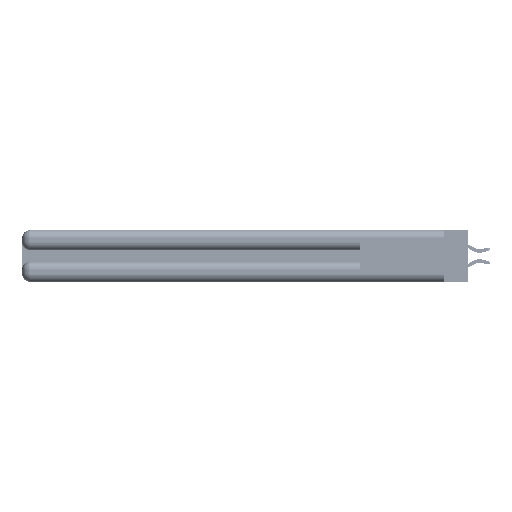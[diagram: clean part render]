
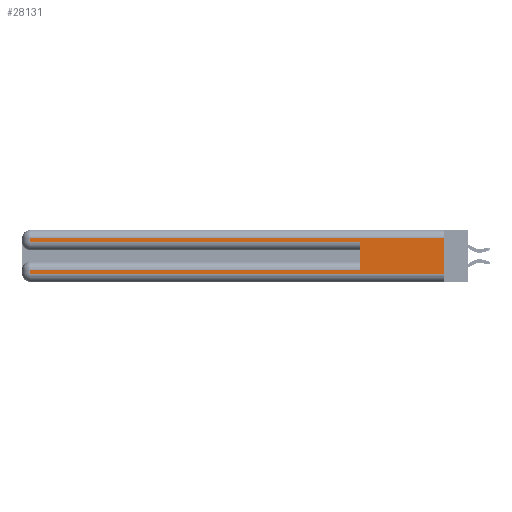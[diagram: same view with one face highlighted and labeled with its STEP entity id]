
A CAD part, left-side view. The second image highlights one B-rep face of the part: STEP entity #28131.
In plain terms, the highlighted planar face has unit normal (-1, 0, 0).
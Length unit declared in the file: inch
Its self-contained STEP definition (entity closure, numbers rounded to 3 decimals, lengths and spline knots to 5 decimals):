
#3 = EDGE_LOOP ( 'NONE', ( #18414, #37219, #32629, #33383, #12969, #47455, #42234, #39631 ) ) ;
#504 = EDGE_CURVE ( 'NONE', #51900, #22637, #47891, .T. ) ;
#625 = VECTOR ( 'NONE', #6461, 39.37008 ) ;
#2067 = LINE ( 'NONE', #34609, #21926 ) ;
#4163 = EDGE_CURVE ( 'NONE', #12128, #20755, #49559, .T. ) ;
#4641 = VECTOR ( 'NONE', #5702, 39.37008 ) ;
#5702 = DIRECTION ( 'NONE',  ( 0., 1., 0. ) ) ;
#6461 = DIRECTION ( 'NONE',  ( 0., 0., -1. ) ) ;
#8053 = EDGE_CURVE ( 'NONE', #45056, #49565, #25386, .T. ) ;
#8858 = CARTESIAN_POINT ( 'NONE',  ( 0., 0.6, 0.285 ) ) ;
#8896 = LINE ( 'NONE', #9161, #18818 ) ;
#9161 = CARTESIAN_POINT ( 'NONE',  ( 0., 2.94, 0.37 ) ) ;
#10229 = CARTESIAN_POINT ( 'NONE',  ( 0., 0., 0.085 ) ) ;
#11843 = CARTESIAN_POINT ( 'NONE',  ( 0., 0., 0.37 ) ) ;
#11967 = LINE ( 'NONE', #36004, #625 ) ;
#12128 = VERTEX_POINT ( 'NONE', #51677 ) ;
#12969 = ORIENTED_EDGE ( 'NONE', *, *, #20425, .F. ) ;
#14030 = EDGE_CURVE ( 'NONE', #29570, #34548, #2067, .T. ) ;
#14033 = CARTESIAN_POINT ( 'NONE',  ( 0., 0., 0.31 ) ) ;
#14409 = CARTESIAN_POINT ( 'NONE',  ( 0., 0.6, 0.145 ) ) ;
#16078 = DIRECTION ( 'NONE',  ( 0., 0., -1. ) ) ;
#16419 = CARTESIAN_POINT ( 'NONE',  ( 0., 2.94, 0.31 ) ) ;
#16891 = FACE_OUTER_BOUND ( 'NONE', #3, .T. ) ;
#17094 = CARTESIAN_POINT ( 'NONE',  ( 0., 0., 0.37 ) ) ;
#18414 = ORIENTED_EDGE ( 'NONE', *, *, #40958, .F. ) ;
#18684 = VECTOR ( 'NONE', #42383, 39.37008 ) ;
#18818 = VECTOR ( 'NONE', #51245, 39.37008 ) ;
#20425 = EDGE_CURVE ( 'NONE', #51900, #49565, #47072, .T. ) ;
#20755 = VERTEX_POINT ( 'NONE', #16419 ) ;
#21815 = CARTESIAN_POINT ( 'NONE',  ( 0., 0., 0.285 ) ) ;
#21926 = VECTOR ( 'NONE', #26096, 39.37008 ) ;
#22637 = VERTEX_POINT ( 'NONE', #32706 ) ;
#24983 = CARTESIAN_POINT ( 'NONE',  ( 0., 2.94, 0.06 ) ) ;
#25046 = CARTESIAN_POINT ( 'NONE',  ( 0., 0., 0.06 ) ) ;
#25386 = LINE ( 'NONE', #21815, #35301 ) ;
#26096 = DIRECTION ( 'NONE',  ( 0., -1., 0. ) ) ;
#26331 = CARTESIAN_POINT ( 'NONE',  ( 0., 0.6, 0.085 ) ) ;
#28131 = ADVANCED_FACE ( 'NONE', ( #16891 ), #37140, .F. ) ;
#29570 = VERTEX_POINT ( 'NONE', #24983 ) ;
#32629 = ORIENTED_EDGE ( 'NONE', *, *, #42019, .T. ) ;
#32706 = CARTESIAN_POINT ( 'NONE',  ( 0., 2.94, 0.085 ) ) ;
#32814 = EDGE_CURVE ( 'NONE', #22637, #29570, #8896, .T. ) ;
#33383 = ORIENTED_EDGE ( 'NONE', *, *, #8053, .T. ) ;
#34548 = VERTEX_POINT ( 'NONE', #25046 ) ;
#34609 = CARTESIAN_POINT ( 'NONE',  ( 0., 0., 0.06 ) ) ;
#35301 = VECTOR ( 'NONE', #43009, 39.37008 ) ;
#35519 = DIRECTION ( 'NONE',  ( 0., 1., 0. ) ) ;
#36004 = CARTESIAN_POINT ( 'NONE',  ( 0., 2.94, 0.37 ) ) ;
#37140 = PLANE ( 'NONE',  #48047 ) ;
#37219 = ORIENTED_EDGE ( 'NONE', *, *, #4163, .T. ) ;
#39631 = ORIENTED_EDGE ( 'NONE', *, *, #14030, .T. ) ;
#40958 = EDGE_CURVE ( 'NONE', #12128, #34548, #41150, .T. ) ;
#41150 = LINE ( 'NONE', #17094, #18684 ) ;
#41269 = CARTESIAN_POINT ( 'NONE',  ( 0., 2.94, 0.285 ) ) ;
#41380 = DIRECTION ( 'NONE',  ( 1., 0., 0. ) ) ;
#42019 = EDGE_CURVE ( 'NONE', #20755, #45056, #11967, .T. ) ;
#42234 = ORIENTED_EDGE ( 'NONE', *, *, #32814, .T. ) ;
#42383 = DIRECTION ( 'NONE',  ( 0., 0., -1. ) ) ;
#43009 = DIRECTION ( 'NONE',  ( 0., -1., 0. ) ) ;
#45056 = VERTEX_POINT ( 'NONE', #41269 ) ;
#45756 = VECTOR ( 'NONE', #48183, 39.37008 ) ;
#47072 = LINE ( 'NONE', #14409, #45756 ) ;
#47455 = ORIENTED_EDGE ( 'NONE', *, *, #504, .T. ) ;
#47891 = LINE ( 'NONE', #10229, #49221 ) ;
#48047 = AXIS2_PLACEMENT_3D ( 'NONE', #11843, #41380, #16078 ) ;
#48183 = DIRECTION ( 'NONE',  ( 0., 0., 1. ) ) ;
#49221 = VECTOR ( 'NONE', #35519, 39.37008 ) ;
#49559 = LINE ( 'NONE', #14033, #4641 ) ;
#49565 = VERTEX_POINT ( 'NONE', #8858 ) ;
#51245 = DIRECTION ( 'NONE',  ( 0., 0., -1. ) ) ;
#51677 = CARTESIAN_POINT ( 'NONE',  ( 0., 0., 0.31 ) ) ;
#51900 = VERTEX_POINT ( 'NONE', #26331 ) ;
